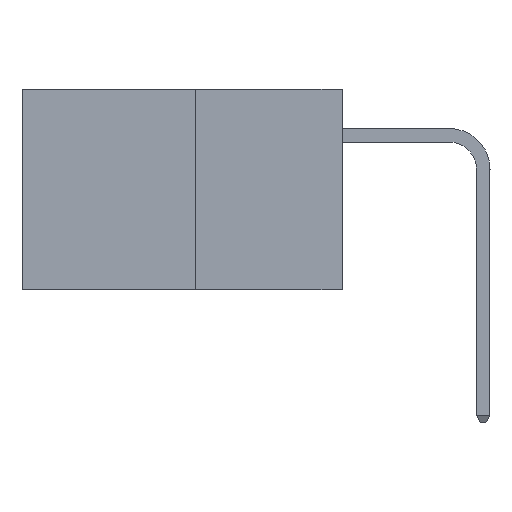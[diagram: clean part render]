
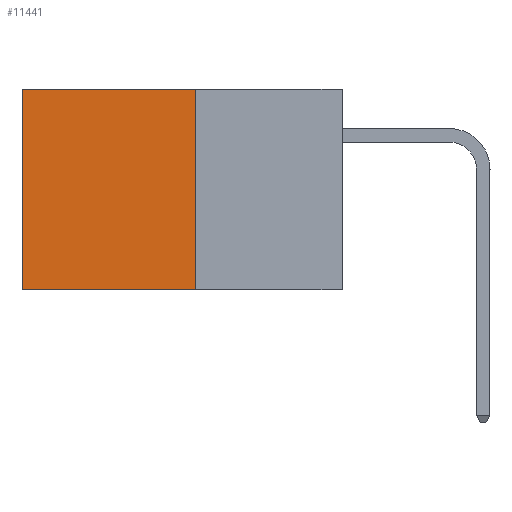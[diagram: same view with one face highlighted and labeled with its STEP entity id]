
A CAD part, left-side view. The second image highlights one B-rep face of the part: STEP entity #11441.
In plain terms, the highlighted planar face has unit normal (-1, 0, 0).
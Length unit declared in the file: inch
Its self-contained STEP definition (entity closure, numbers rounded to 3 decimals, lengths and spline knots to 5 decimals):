
#129 = CARTESIAN_POINT ( 'NONE',  ( 0.277, 0.27, 0. ) ) ;
#731 = ORIENTED_EDGE ( 'NONE', *, *, #9027, .F. ) ;
#755 = ORIENTED_EDGE ( 'NONE', *, *, #3573, .T. ) ;
#1029 = EDGE_LOOP ( 'NONE', ( #11703, #14156, #731, #755 ) ) ;
#1249 = CARTESIAN_POINT ( 'NONE',  ( 0.277, 0.27, -0.37 ) ) ;
#1270 = LINE ( 'NONE', #129, #10617 ) ;
#1299 = DIRECTION ( 'NONE',  ( 0., 1., 0. ) ) ;
#1526 = CARTESIAN_POINT ( 'NONE',  ( 0.277, 0.27, -0.37 ) ) ;
#1781 = CARTESIAN_POINT ( 'NONE',  ( 0.277, 0.27, -0.37 ) ) ;
#3110 = CARTESIAN_POINT ( 'NONE',  ( 0.277, 0.27, -0.37 ) ) ;
#3317 = AXIS2_PLACEMENT_3D ( 'NONE', #3110, #11561, #4321 ) ;
#3573 = EDGE_CURVE ( 'NONE', #6146, #11297, #1270, .T. ) ;
#3942 = LINE ( 'NONE', #1526, #15524 ) ;
#4321 = DIRECTION ( 'NONE',  ( 0., 0., -1. ) ) ;
#4963 = LINE ( 'NONE', #6276, #14883 ) ;
#6146 = VERTEX_POINT ( 'NONE', #7413 ) ;
#6276 = CARTESIAN_POINT ( 'NONE',  ( 0.277, 0.59, -0.37 ) ) ;
#6750 = PLANE ( 'NONE',  #3317 ) ;
#6891 = VERTEX_POINT ( 'NONE', #1249 ) ;
#6905 = FACE_OUTER_BOUND ( 'NONE', #1029, .T. ) ;
#7088 = CARTESIAN_POINT ( 'NONE',  ( 0.277, 0.59, -0.37 ) ) ;
#7190 = VECTOR ( 'NONE', #12669, 39.37008 ) ;
#7413 = CARTESIAN_POINT ( 'NONE',  ( 0.277, 0.27, 0. ) ) ;
#8224 = EDGE_CURVE ( 'NONE', #6891, #11063, #3942, .T. ) ;
#9027 = EDGE_CURVE ( 'NONE', #6146, #6891, #10386, .T. ) ;
#9927 = DIRECTION ( 'NONE',  ( 0., 0., -1. ) ) ;
#10386 = LINE ( 'NONE', #1781, #7190 ) ;
#10617 = VECTOR ( 'NONE', #1299, 39.37008 ) ;
#11063 = VERTEX_POINT ( 'NONE', #7088 ) ;
#11297 = VERTEX_POINT ( 'NONE', #14796 ) ;
#11441 = ADVANCED_FACE ( 'NONE', ( #6905 ), #6750, .F. ) ;
#11561 = DIRECTION ( 'NONE',  ( 1., 0., 0. ) ) ;
#11703 = ORIENTED_EDGE ( 'NONE', *, *, #15444, .T. ) ;
#12435 = DIRECTION ( 'NONE',  ( 0., 1., 0. ) ) ;
#12669 = DIRECTION ( 'NONE',  ( 0., 0., -1. ) ) ;
#14156 = ORIENTED_EDGE ( 'NONE', *, *, #8224, .F. ) ;
#14796 = CARTESIAN_POINT ( 'NONE',  ( 0.277, 0.59, 0. ) ) ;
#14883 = VECTOR ( 'NONE', #9927, 39.37008 ) ;
#15444 = EDGE_CURVE ( 'NONE', #11297, #11063, #4963, .T. ) ;
#15524 = VECTOR ( 'NONE', #12435, 39.37008 ) ;
